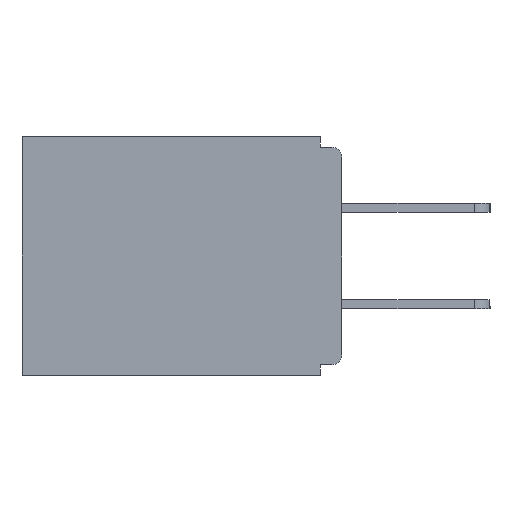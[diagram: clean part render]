
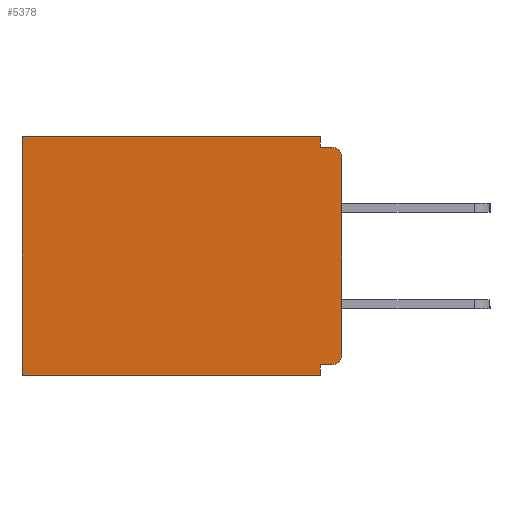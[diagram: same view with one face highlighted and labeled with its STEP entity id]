
A CAD part, left-side view. The second image highlights one B-rep face of the part: STEP entity #5378.
In plain terms, the highlighted planar face has unit normal (-1, 0, 0).
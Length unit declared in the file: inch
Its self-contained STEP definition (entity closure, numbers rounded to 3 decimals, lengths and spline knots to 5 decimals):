
#180 = DIRECTION ( 'NONE',  ( -1., 0., 0. ) ) ;
#662 = CARTESIAN_POINT ( 'NONE',  ( 0.298, 0.46, 0. ) ) ;
#1202 = EDGE_CURVE ( 'NONE', #23721, #11305, #15935, .T. ) ;
#1433 = CARTESIAN_POINT ( 'NONE',  ( 0.298, 0., 0. ) ) ;
#2378 = DIRECTION ( 'NONE',  ( 0., 0., -1. ) ) ;
#2438 = ORIENTED_EDGE ( 'NONE', *, *, #8735, .T. ) ;
#2594 = LINE ( 'NONE', #17473, #7924 ) ;
#2905 = VERTEX_POINT ( 'NONE', #10545 ) ;
#3656 = CIRCLE ( 'NONE', #9267, 0.015 ) ;
#3990 = CARTESIAN_POINT ( 'NONE',  ( 0.298, 0.46, 0. ) ) ;
#4130 = VECTOR ( 'NONE', #11669, 39.37008 ) ;
#4254 = EDGE_CURVE ( 'NONE', #20818, #2905, #4570, .T. ) ;
#4570 = LINE ( 'NONE', #15498, #16634 ) ;
#4704 = DIRECTION ( 'NONE',  ( 0., 0., -1. ) ) ;
#5313 = VECTOR ( 'NONE', #12541, 39.37008 ) ;
#5378 = ADVANCED_FACE ( 'NONE', ( #8844 ), #5839, .F. ) ;
#5699 = VERTEX_POINT ( 'NONE', #24183 ) ;
#5735 = DIRECTION ( 'NONE',  ( 1., 0., 0. ) ) ;
#5839 = PLANE ( 'NONE',  #23268 ) ;
#6277 = DIRECTION ( 'NONE',  ( 0., 0., -1. ) ) ;
#6301 = ORIENTED_EDGE ( 'NONE', *, *, #6330, .F. ) ;
#6330 = EDGE_CURVE ( 'NONE', #21785, #5699, #23903, .T. ) ;
#6382 = ORIENTED_EDGE ( 'NONE', *, *, #24430, .F. ) ;
#7107 = CARTESIAN_POINT ( 'NONE',  ( 0.298, 0.031, -0.015 ) ) ;
#7479 = DIRECTION ( 'NONE',  ( -1., 0., 0. ) ) ;
#7492 = CARTESIAN_POINT ( 'NONE',  ( 0.298, 0., -0.343 ) ) ;
#7724 = VERTEX_POINT ( 'NONE', #24173 ) ;
#7906 = LINE ( 'NONE', #662, #20987 ) ;
#7924 = VECTOR ( 'NONE', #21771, 39.37008 ) ;
#7970 = DIRECTION ( 'NONE',  ( 0., 0., -1. ) ) ;
#8254 = EDGE_CURVE ( 'NONE', #23721, #5699, #3656, .T. ) ;
#8424 = CARTESIAN_POINT ( 'NONE',  ( 0.298, 0.031, -0.328 ) ) ;
#8735 = EDGE_CURVE ( 'NONE', #7724, #10059, #11001, .T. ) ;
#8844 = FACE_OUTER_BOUND ( 'NONE', #27138, .T. ) ;
#9267 = AXIS2_PLACEMENT_3D ( 'NONE', #17609, #180, #15264 ) ;
#9423 = LINE ( 'NONE', #21863, #27551 ) ;
#9908 = VERTEX_POINT ( 'NONE', #14137 ) ;
#10059 = VERTEX_POINT ( 'NONE', #3990 ) ;
#10545 = CARTESIAN_POINT ( 'NONE',  ( 0.298, 0.015, -0.015 ) ) ;
#11001 = LINE ( 'NONE', #18804, #5313 ) ;
#11109 = AXIS2_PLACEMENT_3D ( 'NONE', #19116, #7479, #6277 ) ;
#11305 = VERTEX_POINT ( 'NONE', #8424 ) ;
#11587 = VECTOR ( 'NONE', #19012, 39.37008 ) ;
#11669 = DIRECTION ( 'NONE',  ( 0., 0., -1. ) ) ;
#12412 = CARTESIAN_POINT ( 'NONE',  ( 0.298, 0., -0.03 ) ) ;
#12541 = DIRECTION ( 'NONE',  ( 0., 1., 0. ) ) ;
#13244 = ORIENTED_EDGE ( 'NONE', *, *, #8254, .T. ) ;
#13465 = CARTESIAN_POINT ( 'NONE',  ( 0.298, 0., 0. ) ) ;
#14137 = CARTESIAN_POINT ( 'NONE',  ( 0.298, 0.031, -0.343 ) ) ;
#14146 = EDGE_CURVE ( 'NONE', #9908, #18246, #19152, .T. ) ;
#14695 = ORIENTED_EDGE ( 'NONE', *, *, #27563, .F. ) ;
#15264 = DIRECTION ( 'NONE',  ( 0., 0., -1. ) ) ;
#15403 = DIRECTION ( 'NONE',  ( 0., -1., 0. ) ) ;
#15498 = CARTESIAN_POINT ( 'NONE',  ( 0.298, 0., -0.015 ) ) ;
#15935 = LINE ( 'NONE', #19392, #11587 ) ;
#16114 = VECTOR ( 'NONE', #18109, 39.37008 ) ;
#16634 = VECTOR ( 'NONE', #15403, 39.37008 ) ;
#17236 = ORIENTED_EDGE ( 'NONE', *, *, #22429, .T. ) ;
#17473 = CARTESIAN_POINT ( 'NONE',  ( 0.298, 0.031, -0.343 ) ) ;
#17609 = CARTESIAN_POINT ( 'NONE',  ( 0.298, 0.015, -0.313 ) ) ;
#18109 = DIRECTION ( 'NONE',  ( 0., 1., 0. ) ) ;
#18246 = VERTEX_POINT ( 'NONE', #20055 ) ;
#18804 = CARTESIAN_POINT ( 'NONE',  ( 0.298, 0., 0. ) ) ;
#19012 = DIRECTION ( 'NONE',  ( 0., 1., 0. ) ) ;
#19116 = CARTESIAN_POINT ( 'NONE',  ( 0.298, 0.015, -0.03 ) ) ;
#19152 = LINE ( 'NONE', #7492, #16114 ) ;
#19392 = CARTESIAN_POINT ( 'NONE',  ( 0.298, 0., -0.328 ) ) ;
#20055 = CARTESIAN_POINT ( 'NONE',  ( 0.298, 0.46, -0.343 ) ) ;
#20818 = VERTEX_POINT ( 'NONE', #7107 ) ;
#20973 = EDGE_CURVE ( 'NONE', #10059, #18246, #7906, .T. ) ;
#20987 = VECTOR ( 'NONE', #4704, 39.37008 ) ;
#21235 = ORIENTED_EDGE ( 'NONE', *, *, #4254, .F. ) ;
#21425 = CARTESIAN_POINT ( 'NONE',  ( 0.298, 0.015, -0.328 ) ) ;
#21771 = DIRECTION ( 'NONE',  ( 0., 0., -1. ) ) ;
#21783 = ORIENTED_EDGE ( 'NONE', *, *, #14146, .F. ) ;
#21785 = VERTEX_POINT ( 'NONE', #12412 ) ;
#21863 = CARTESIAN_POINT ( 'NONE',  ( 0.298, 0.031, -0.343 ) ) ;
#22429 = EDGE_CURVE ( 'NONE', #21785, #2905, #27190, .T. ) ;
#23268 = AXIS2_PLACEMENT_3D ( 'NONE', #1433, #5735, #7970 ) ;
#23522 = ORIENTED_EDGE ( 'NONE', *, *, #20973, .T. ) ;
#23721 = VERTEX_POINT ( 'NONE', #21425 ) ;
#23903 = LINE ( 'NONE', #13465, #4130 ) ;
#24173 = CARTESIAN_POINT ( 'NONE',  ( 0.298, 0.031, 0. ) ) ;
#24183 = CARTESIAN_POINT ( 'NONE',  ( 0.298, 0., -0.313 ) ) ;
#24348 = ORIENTED_EDGE ( 'NONE', *, *, #1202, .F. ) ;
#24430 = EDGE_CURVE ( 'NONE', #7724, #20818, #2594, .T. ) ;
#27138 = EDGE_LOOP ( 'NONE', ( #17236, #21235, #6382, #2438, #23522, #21783, #14695, #24348, #13244, #6301 ) ) ;
#27190 = CIRCLE ( 'NONE', #11109, 0.015 ) ;
#27551 = VECTOR ( 'NONE', #2378, 39.37008 ) ;
#27563 = EDGE_CURVE ( 'NONE', #11305, #9908, #9423, .T. ) ;
